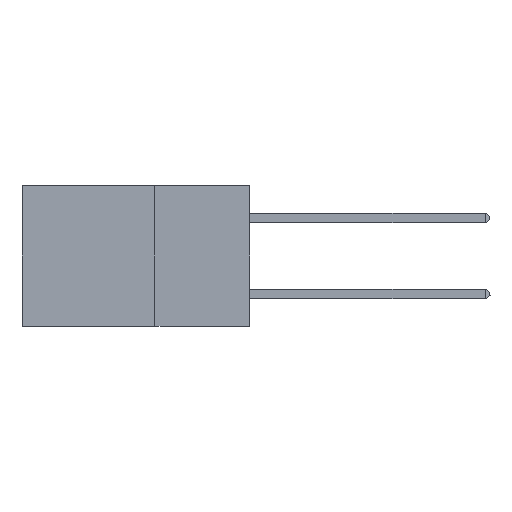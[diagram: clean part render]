
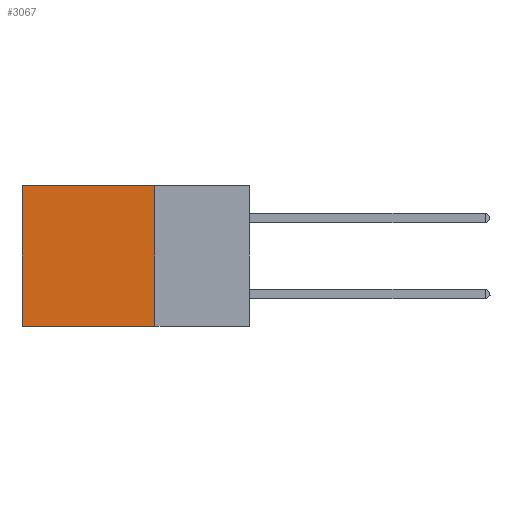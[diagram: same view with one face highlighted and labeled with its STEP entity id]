
A CAD part, left-side view. The second image highlights one B-rep face of the part: STEP entity #3067.
In plain terms, the highlighted planar face has unit normal (-1, 0, 0).
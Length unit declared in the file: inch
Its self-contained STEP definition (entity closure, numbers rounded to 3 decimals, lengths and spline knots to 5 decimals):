
#20 = ORIENTED_EDGE ( 'NONE', *, *, #8356, .T. ) ;
#257 = VECTOR ( 'NONE', #2561, 39.37008 ) ;
#458 = CARTESIAN_POINT ( 'NONE',  ( 0.2875, 0.25, 0. ) ) ;
#1832 = ORIENTED_EDGE ( 'NONE', *, *, #16537, .F. ) ;
#2143 = CARTESIAN_POINT ( 'NONE',  ( 0.2875, 0.25, 0. ) ) ;
#2561 = DIRECTION ( 'NONE',  ( 0., 0., -1. ) ) ;
#2570 = EDGE_CURVE ( 'NONE', #6406, #8896, #12540, .T. ) ;
#3067 = ADVANCED_FACE ( 'NONE', ( #11260 ), #11206, .F. ) ;
#3988 = CARTESIAN_POINT ( 'NONE',  ( 0.2875, 0.25, 0. ) ) ;
#4532 = DIRECTION ( 'NONE',  ( 0., 0., -1. ) ) ;
#5419 = VECTOR ( 'NONE', #14113, 39.37008 ) ;
#6148 = DIRECTION ( 'NONE',  ( 0., 1., 0. ) ) ;
#6406 = VERTEX_POINT ( 'NONE', #14400 ) ;
#6982 = LINE ( 'NONE', #10499, #257 ) ;
#8356 = EDGE_CURVE ( 'NONE', #10430, #8896, #6982, .T. ) ;
#8763 = CARTESIAN_POINT ( 'NONE',  ( 0.2875, 0.25, -0.37 ) ) ;
#8896 = VERTEX_POINT ( 'NONE', #10305 ) ;
#9466 = EDGE_CURVE ( 'NONE', #11072, #10430, #14729, .T. ) ;
#10305 = CARTESIAN_POINT ( 'NONE',  ( 0.2875, 0.6, -0.37 ) ) ;
#10430 = VERTEX_POINT ( 'NONE', #14744 ) ;
#10499 = CARTESIAN_POINT ( 'NONE',  ( 0.2875, 0.6, 0. ) ) ;
#10586 = VECTOR ( 'NONE', #14734, 39.37008 ) ;
#11072 = VERTEX_POINT ( 'NONE', #14347 ) ;
#11206 = PLANE ( 'NONE',  #11837 ) ;
#11260 = FACE_OUTER_BOUND ( 'NONE', #13995, .T. ) ;
#11753 = ORIENTED_EDGE ( 'NONE', *, *, #2570, .F. ) ;
#11837 = AXIS2_PLACEMENT_3D ( 'NONE', #458, #12558, #4532 ) ;
#12540 = LINE ( 'NONE', #8763, #5419 ) ;
#12558 = DIRECTION ( 'NONE',  ( 1., 0., 0. ) ) ;
#12905 = ORIENTED_EDGE ( 'NONE', *, *, #9466, .T. ) ;
#13995 = EDGE_LOOP ( 'NONE', ( #20, #11753, #1832, #12905 ) ) ;
#14113 = DIRECTION ( 'NONE',  ( 0., 1., 0. ) ) ;
#14161 = LINE ( 'NONE', #3988, #10586 ) ;
#14306 = VECTOR ( 'NONE', #6148, 39.37008 ) ;
#14347 = CARTESIAN_POINT ( 'NONE',  ( 0.2875, 0.25, 0. ) ) ;
#14400 = CARTESIAN_POINT ( 'NONE',  ( 0.2875, 0.25, -0.37 ) ) ;
#14729 = LINE ( 'NONE', #2143, #14306 ) ;
#14734 = DIRECTION ( 'NONE',  ( 0., 0., -1. ) ) ;
#14744 = CARTESIAN_POINT ( 'NONE',  ( 0.2875, 0.6, 0. ) ) ;
#16537 = EDGE_CURVE ( 'NONE', #11072, #6406, #14161, .T. ) ;
